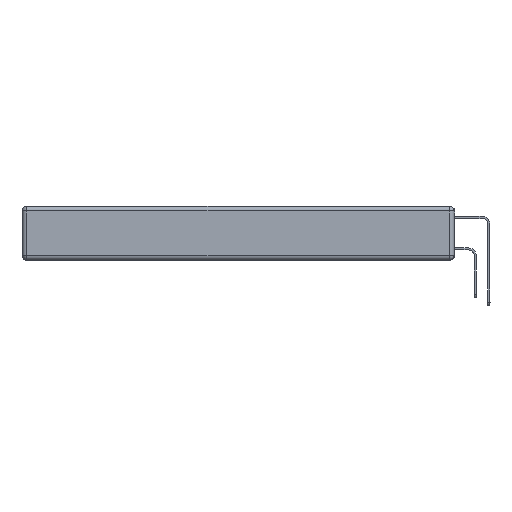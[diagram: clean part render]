
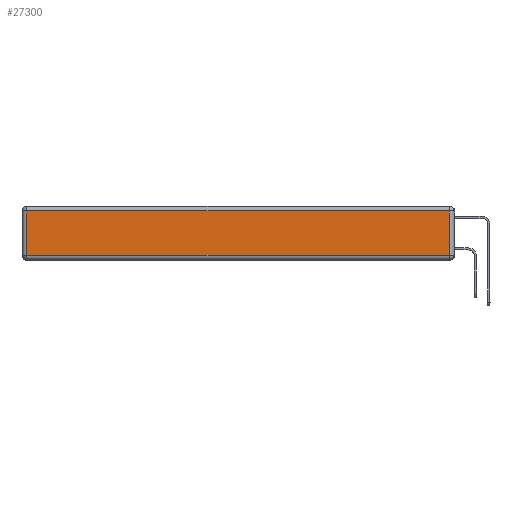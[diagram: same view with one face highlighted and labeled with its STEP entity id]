
A CAD part, left-side view. The second image highlights one B-rep face of the part: STEP entity #27300.
In plain terms, the highlighted planar face has unit normal (-1, 0, 0).
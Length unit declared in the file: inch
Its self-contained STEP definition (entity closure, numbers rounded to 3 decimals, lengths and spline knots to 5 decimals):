
#9 = DIRECTION ( 'NONE',  ( 0., 0., 1. ) ) ;
#1671 = LINE ( 'NONE', #20088, #16451 ) ;
#4463 = DIRECTION ( 'NONE',  ( -1., 0., 0. ) ) ;
#6420 = EDGE_CURVE ( 'NONE', #16583, #11387, #1671, .T. ) ;
#6897 = ORIENTED_EDGE ( 'NONE', *, *, #9093, .T. ) ;
#7039 = CARTESIAN_POINT ( 'NONE',  ( 0., 2.75, -0.03 ) ) ;
#7089 = CARTESIAN_POINT ( 'NONE',  ( 0., 0.03, -0.03 ) ) ;
#7188 = DIRECTION ( 'NONE',  ( 0., 1., 0. ) ) ;
#8671 = AXIS2_PLACEMENT_3D ( 'NONE', #25602, #4463, #9 ) ;
#9093 = EDGE_CURVE ( 'NONE', #11387, #20307, #27647, .T. ) ;
#9384 = VECTOR ( 'NONE', #25067, 39.37008 ) ;
#10028 = LINE ( 'NONE', #10463, #29594 ) ;
#10463 = CARTESIAN_POINT ( 'NONE',  ( 0., 0.03, -0.343 ) ) ;
#11387 = VERTEX_POINT ( 'NONE', #25299 ) ;
#11435 = EDGE_CURVE ( 'NONE', #14480, #16583, #18586, .T. ) ;
#14480 = VERTEX_POINT ( 'NONE', #7089 ) ;
#15866 = VECTOR ( 'NONE', #7188, 39.37008 ) ;
#15922 = CARTESIAN_POINT ( 'NONE',  ( 0., 0., -0.313 ) ) ;
#16451 = VECTOR ( 'NONE', #17799, 39.37008 ) ;
#16583 = VERTEX_POINT ( 'NONE', #17679 ) ;
#17679 = CARTESIAN_POINT ( 'NONE',  ( 0., 2.72, -0.03 ) ) ;
#17799 = DIRECTION ( 'NONE',  ( 0., 0., -1. ) ) ;
#18586 = LINE ( 'NONE', #7039, #15866 ) ;
#19455 = DIRECTION ( 'NONE',  ( 0., 0., 1. ) ) ;
#20088 = CARTESIAN_POINT ( 'NONE',  ( 0., 2.72, -0.343 ) ) ;
#20307 = VERTEX_POINT ( 'NONE', #26565 ) ;
#20816 = ORIENTED_EDGE ( 'NONE', *, *, #6420, .T. ) ;
#23004 = PLANE ( 'NONE',  #8671 ) ;
#24090 = EDGE_LOOP ( 'NONE', ( #6897, #25775, #29754, #20816 ) ) ;
#25067 = DIRECTION ( 'NONE',  ( 0., -1., 0. ) ) ;
#25299 = CARTESIAN_POINT ( 'NONE',  ( 0., 2.72, -0.313 ) ) ;
#25602 = CARTESIAN_POINT ( 'NONE',  ( 0., 0., -0.343 ) ) ;
#25759 = FACE_OUTER_BOUND ( 'NONE', #24090, .T. ) ;
#25775 = ORIENTED_EDGE ( 'NONE', *, *, #29757, .T. ) ;
#26565 = CARTESIAN_POINT ( 'NONE',  ( 0., 0.03, -0.313 ) ) ;
#27300 = ADVANCED_FACE ( 'NONE', ( #25759 ), #23004, .T. ) ;
#27647 = LINE ( 'NONE', #15922, #9384 ) ;
#29594 = VECTOR ( 'NONE', #19455, 39.37008 ) ;
#29754 = ORIENTED_EDGE ( 'NONE', *, *, #11435, .T. ) ;
#29757 = EDGE_CURVE ( 'NONE', #20307, #14480, #10028, .T. ) ;
